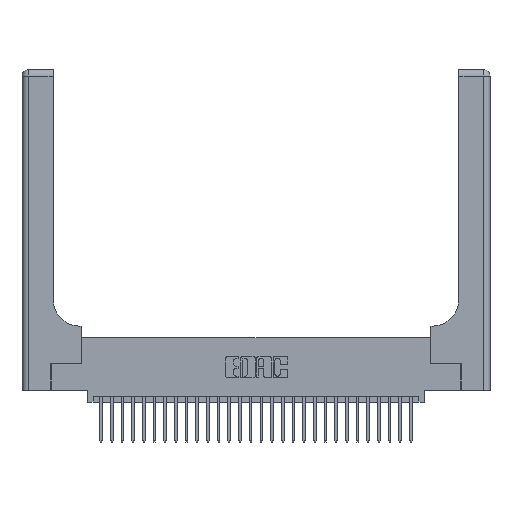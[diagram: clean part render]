
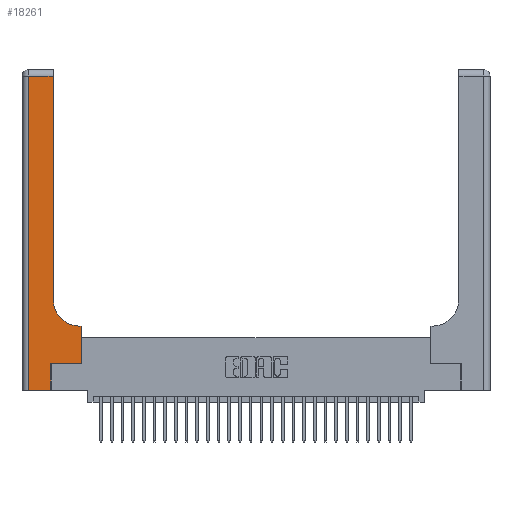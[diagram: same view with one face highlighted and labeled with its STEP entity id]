
A CAD part, top view. The second image highlights one B-rep face of the part: STEP entity #18261.
In plain terms, the highlighted planar face has unit normal (0, 0, 1).
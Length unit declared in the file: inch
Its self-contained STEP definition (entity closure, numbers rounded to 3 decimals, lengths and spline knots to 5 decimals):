
#457 = VERTEX_POINT ( 'NONE', #21394 ) ;
#680 = ORIENTED_EDGE ( 'NONE', *, *, #2590, .T. ) ;
#970 = VERTEX_POINT ( 'NONE', #4604 ) ;
#1414 = ORIENTED_EDGE ( 'NONE', *, *, #15162, .T. ) ;
#2070 = PLANE ( 'NONE',  #21146 ) ;
#2590 = EDGE_CURVE ( 'NONE', #457, #7942, #27687, .T. ) ;
#2615 = ORIENTED_EDGE ( 'NONE', *, *, #7205, .T. ) ;
#3012 = EDGE_CURVE ( 'NONE', #14626, #16128, #4900, .T. ) ;
#4451 = ORIENTED_EDGE ( 'NONE', *, *, #29347, .T. ) ;
#4488 = DIRECTION ( 'NONE',  ( -1., 0., 0. ) ) ;
#4550 = DIRECTION ( 'NONE',  ( 0., 0., -1. ) ) ;
#4604 = CARTESIAN_POINT ( 'NONE',  ( 0.2915, 2.94, 0.37 ) ) ;
#4705 = EDGE_CURVE ( 'NONE', #7942, #30449, #16693, .T. ) ;
#4900 = CIRCLE ( 'NONE', #23205, 0.25 ) ;
#5041 = DIRECTION ( 'NONE',  ( 1., 0., 0. ) ) ;
#6155 = EDGE_CURVE ( 'NONE', #12155, #457, #29003, .T. ) ;
#7205 = EDGE_CURVE ( 'NONE', #12878, #12155, #9784, .T. ) ;
#7857 = CARTESIAN_POINT ( 'NONE',  ( 0.06, 2.94, 0.37 ) ) ;
#7942 = VERTEX_POINT ( 'NONE', #11325 ) ;
#8046 = ORIENTED_EDGE ( 'NONE', *, *, #10163, .T. ) ;
#8993 = VECTOR ( 'NONE', #14749, 39.37008 ) ;
#9784 = LINE ( 'NONE', #20404, #21542 ) ;
#9865 = CARTESIAN_POINT ( 'NONE',  ( 0.06, 0., 0.37 ) ) ;
#9929 = VECTOR ( 'NONE', #27933, 39.37008 ) ;
#10163 = EDGE_CURVE ( 'NONE', #16128, #970, #26509, .T. ) ;
#10683 = LINE ( 'NONE', #20911, #9929 ) ;
#11325 = CARTESIAN_POINT ( 'NONE',  ( 0.269, 0.25, 0.37 ) ) ;
#12152 = ORIENTED_EDGE ( 'NONE', *, *, #3012, .T. ) ;
#12155 = VERTEX_POINT ( 'NONE', #9865 ) ;
#12353 = CARTESIAN_POINT ( 'NONE',  ( 0.269, 0., 0.37 ) ) ;
#12878 = VERTEX_POINT ( 'NONE', #7857 ) ;
#12882 = EDGE_CURVE ( 'NONE', #16195, #14626, #28895, .T. ) ;
#13811 = ORIENTED_EDGE ( 'NONE', *, *, #4705, .T. ) ;
#14102 = VECTOR ( 'NONE', #14319, 39.37008 ) ;
#14319 = DIRECTION ( 'NONE',  ( 0., 1., 0. ) ) ;
#14626 = VERTEX_POINT ( 'NONE', #19008 ) ;
#14749 = DIRECTION ( 'NONE',  ( 0., 1., 0. ) ) ;
#15027 = DIRECTION ( 'NONE',  ( -1., 0., 0. ) ) ;
#15162 = EDGE_CURVE ( 'NONE', #970, #12878, #10683, .T. ) ;
#16128 = VERTEX_POINT ( 'NONE', #21910 ) ;
#16193 = CARTESIAN_POINT ( 'NONE',  ( 0., 3., 0.37 ) ) ;
#16195 = VERTEX_POINT ( 'NONE', #26775 ) ;
#16197 = EDGE_LOOP ( 'NONE', ( #8046, #1414, #2615, #18040, #680, #13811, #4451, #27980, #12152 ) ) ;
#16509 = DIRECTION ( 'NONE',  ( 1., 0., 0. ) ) ;
#16693 = LINE ( 'NONE', #25737, #28359 ) ;
#18040 = ORIENTED_EDGE ( 'NONE', *, *, #6155, .T. ) ;
#18261 = ADVANCED_FACE ( 'NONE', ( #26572 ), #2070, .F. ) ;
#18635 = DIRECTION ( 'NONE',  ( 0., 0., -1. ) ) ;
#18694 = CARTESIAN_POINT ( 'NONE',  ( 0.5415, 0.85, 0.37 ) ) ;
#19008 = CARTESIAN_POINT ( 'NONE',  ( 0.5415, 0.6, 0.37 ) ) ;
#19521 = CARTESIAN_POINT ( 'NONE',  ( 0.5585, 0.25, 0.37 ) ) ;
#20110 = VECTOR ( 'NONE', #24181, 39.37008 ) ;
#20404 = CARTESIAN_POINT ( 'NONE',  ( 0.06, 3., 0.37 ) ) ;
#20911 = CARTESIAN_POINT ( 'NONE',  ( 0., 2.94, 0.37 ) ) ;
#21037 = DIRECTION ( 'NONE',  ( 1., 0., 0. ) ) ;
#21146 = AXIS2_PLACEMENT_3D ( 'NONE', #16193, #18635, #4488 ) ;
#21382 = CARTESIAN_POINT ( 'NONE',  ( 0.5585, 0.25, 0.37 ) ) ;
#21394 = CARTESIAN_POINT ( 'NONE',  ( 0.269, 0., 0.37 ) ) ;
#21542 = VECTOR ( 'NONE', #22733, 39.37008 ) ;
#21910 = CARTESIAN_POINT ( 'NONE',  ( 0.2915, 0.85, 0.37 ) ) ;
#22065 = VECTOR ( 'NONE', #5041, 39.37008 ) ;
#22682 = VECTOR ( 'NONE', #15027, 39.37008 ) ;
#22733 = DIRECTION ( 'NONE',  ( 0., -1., 0. ) ) ;
#23205 = AXIS2_PLACEMENT_3D ( 'NONE', #18694, #4550, #21037 ) ;
#24181 = DIRECTION ( 'NONE',  ( 0., 1., 0. ) ) ;
#24264 = CARTESIAN_POINT ( 'NONE',  ( 0.2915, 0.6, 0.37 ) ) ;
#25540 = LINE ( 'NONE', #19521, #20110 ) ;
#25737 = CARTESIAN_POINT ( 'NONE',  ( 0.269, 0.25, 0.37 ) ) ;
#26186 = CARTESIAN_POINT ( 'NONE',  ( 0., 0., 0.37 ) ) ;
#26509 = LINE ( 'NONE', #28296, #14102 ) ;
#26572 = FACE_OUTER_BOUND ( 'NONE', #16197, .T. ) ;
#26775 = CARTESIAN_POINT ( 'NONE',  ( 0.5585, 0.6, 0.37 ) ) ;
#27687 = LINE ( 'NONE', #12353, #8993 ) ;
#27933 = DIRECTION ( 'NONE',  ( -1., 0., 0. ) ) ;
#27980 = ORIENTED_EDGE ( 'NONE', *, *, #12882, .T. ) ;
#28296 = CARTESIAN_POINT ( 'NONE',  ( 0.2915, 3., 0.37 ) ) ;
#28359 = VECTOR ( 'NONE', #16509, 39.37008 ) ;
#28895 = LINE ( 'NONE', #24264, #22682 ) ;
#29003 = LINE ( 'NONE', #26186, #22065 ) ;
#29347 = EDGE_CURVE ( 'NONE', #30449, #16195, #25540, .T. ) ;
#30449 = VERTEX_POINT ( 'NONE', #21382 ) ;
